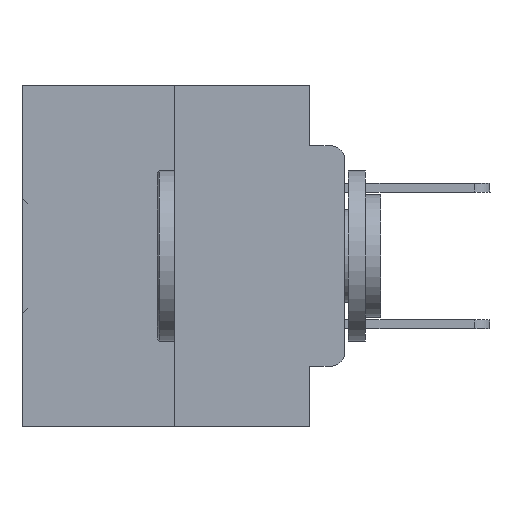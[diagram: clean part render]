
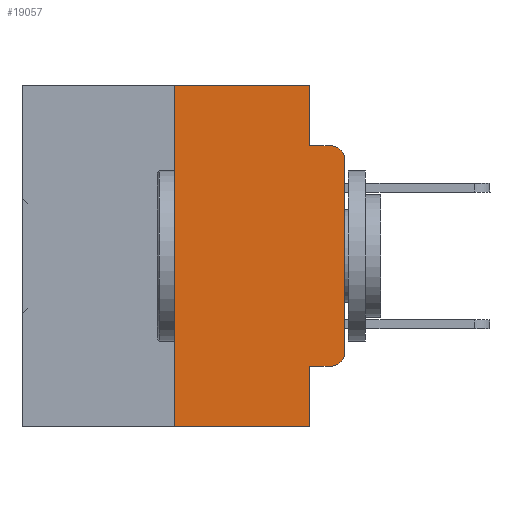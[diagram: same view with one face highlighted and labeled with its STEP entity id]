
A CAD part, left-side view. The second image highlights one B-rep face of the part: STEP entity #19057.
In plain terms, the highlighted planar face has unit normal (-1, 0, 0).
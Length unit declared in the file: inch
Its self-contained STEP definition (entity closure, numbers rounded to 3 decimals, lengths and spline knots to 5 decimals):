
#439 = CARTESIAN_POINT ( 'NONE',  ( 0., 0.25, -0.5 ) ) ;
#452 = VERTEX_POINT ( 'NONE', #18065 ) ;
#732 = LINE ( 'NONE', #26231, #28675 ) ;
#845 = DIRECTION ( 'NONE',  ( 0., 0., -1. ) ) ;
#938 = VERTEX_POINT ( 'NONE', #26433 ) ;
#1768 = EDGE_CURVE ( 'NONE', #10953, #12794, #3225, .T. ) ;
#1987 = ORIENTED_EDGE ( 'NONE', *, *, #24835, .T. ) ;
#2397 = CARTESIAN_POINT ( 'NONE',  ( 0., 0., -0.3915 ) ) ;
#2568 = VECTOR ( 'NONE', #14747, 39.37008 ) ;
#2595 = CARTESIAN_POINT ( 'NONE',  ( 0., 0.051, 0. ) ) ;
#3184 = LINE ( 'NONE', #2595, #34208 ) ;
#3225 = CIRCLE ( 'NONE', #23362, 0.02 ) ;
#3363 = ORIENTED_EDGE ( 'NONE', *, *, #1768, .T. ) ;
#3644 = EDGE_CURVE ( 'NONE', #938, #452, #19149, .T. ) ;
#4663 = EDGE_CURVE ( 'NONE', #452, #25880, #732, .T. ) ;
#4919 = DIRECTION ( 'NONE',  ( 0., 0., -1. ) ) ;
#5444 = EDGE_LOOP ( 'NONE', ( #15345, #13133, #7458, #34054, #29395, #20109, #1987, #13547, #15933, #3363 ) ) ;
#5489 = DIRECTION ( 'NONE',  ( 0., -1., 0. ) ) ;
#5684 = CARTESIAN_POINT ( 'NONE',  ( 0., 0.02, -0.1085 ) ) ;
#6436 = VECTOR ( 'NONE', #14248, 39.37008 ) ;
#6572 = CARTESIAN_POINT ( 'NONE',  ( 0., 0.02, -0.0885 ) ) ;
#7030 = VECTOR ( 'NONE', #5489, 39.37008 ) ;
#7458 = ORIENTED_EDGE ( 'NONE', *, *, #33987, .F. ) ;
#8885 = EDGE_CURVE ( 'NONE', #12794, #18100, #31506, .T. ) ;
#8930 = VERTEX_POINT ( 'NONE', #439 ) ;
#9142 = CIRCLE ( 'NONE', #29656, 0.02 ) ;
#10180 = CARTESIAN_POINT ( 'NONE',  ( 0., 0.051, -0.5 ) ) ;
#10953 = VERTEX_POINT ( 'NONE', #29867 ) ;
#11678 = DIRECTION ( 'NONE',  ( -1., 0., 0. ) ) ;
#11704 = VECTOR ( 'NONE', #27401, 39.37008 ) ;
#11819 = LINE ( 'NONE', #31291, #15779 ) ;
#12794 = VERTEX_POINT ( 'NONE', #2397 ) ;
#12837 = DIRECTION ( 'NONE',  ( -1., 0., 0. ) ) ;
#13133 = ORIENTED_EDGE ( 'NONE', *, *, #15701, .T. ) ;
#13547 = ORIENTED_EDGE ( 'NONE', *, *, #31042, .F. ) ;
#13794 = DIRECTION ( 'NONE',  ( 0., 0., 1. ) ) ;
#14150 = DIRECTION ( 'NONE',  ( 0., -1., 0. ) ) ;
#14248 = DIRECTION ( 'NONE',  ( 0., -1., 0. ) ) ;
#14505 = LINE ( 'NONE', #25138, #7030 ) ;
#14747 = DIRECTION ( 'NONE',  ( 0., 0., 1. ) ) ;
#15257 = VERTEX_POINT ( 'NONE', #6572 ) ;
#15345 = ORIENTED_EDGE ( 'NONE', *, *, #8885, .T. ) ;
#15427 = EDGE_CURVE ( 'NONE', #8930, #938, #20484, .T. ) ;
#15645 = DIRECTION ( 'NONE',  ( 0., 0., -1. ) ) ;
#15701 = EDGE_CURVE ( 'NONE', #18100, #15257, #9142, .T. ) ;
#15779 = VECTOR ( 'NONE', #14150, 39.37008 ) ;
#15933 = ORIENTED_EDGE ( 'NONE', *, *, #23652, .T. ) ;
#15951 = CARTESIAN_POINT ( 'NONE',  ( 0., 0.051, -0.0885 ) ) ;
#17008 = DIRECTION ( 'NONE',  ( 1., 0., 0. ) ) ;
#17283 = DIRECTION ( 'NONE',  ( 0., 0., -1. ) ) ;
#17371 = DIRECTION ( 'NONE',  ( 0., 0., -1. ) ) ;
#17821 = LINE ( 'NONE', #33832, #6436 ) ;
#18065 = CARTESIAN_POINT ( 'NONE',  ( 0., 0.051, 0. ) ) ;
#18100 = VERTEX_POINT ( 'NONE', #32677 ) ;
#19057 = ADVANCED_FACE ( 'NONE', ( #33786 ), #33944, .F. ) ;
#19149 = LINE ( 'NONE', #33002, #11704 ) ;
#20065 = CARTESIAN_POINT ( 'NONE',  ( 0., 0.051, -0.4115 ) ) ;
#20109 = ORIENTED_EDGE ( 'NONE', *, *, #15427, .F. ) ;
#20484 = LINE ( 'NONE', #30232, #28336 ) ;
#22487 = CARTESIAN_POINT ( 'NONE',  ( 0., 0.473, 0. ) ) ;
#23362 = AXIS2_PLACEMENT_3D ( 'NONE', #26730, #12837, #15645 ) ;
#23652 = EDGE_CURVE ( 'NONE', #29158, #10953, #11819, .T. ) ;
#24835 = EDGE_CURVE ( 'NONE', #8930, #31893, #17821, .T. ) ;
#25138 = CARTESIAN_POINT ( 'NONE',  ( 0., 0.051, -0.0885 ) ) ;
#25440 = CARTESIAN_POINT ( 'NONE',  ( 0., 0., 0. ) ) ;
#25880 = VERTEX_POINT ( 'NONE', #15951 ) ;
#26231 = CARTESIAN_POINT ( 'NONE',  ( 0., 0.051, 0. ) ) ;
#26433 = CARTESIAN_POINT ( 'NONE',  ( 0., 0.25, 0. ) ) ;
#26730 = CARTESIAN_POINT ( 'NONE',  ( 0., 0.02, -0.3915 ) ) ;
#27401 = DIRECTION ( 'NONE',  ( 0., -1., 0. ) ) ;
#28336 = VECTOR ( 'NONE', #13794, 39.37008 ) ;
#28675 = VECTOR ( 'NONE', #845, 39.37008 ) ;
#29158 = VERTEX_POINT ( 'NONE', #20065 ) ;
#29395 = ORIENTED_EDGE ( 'NONE', *, *, #3644, .F. ) ;
#29498 = AXIS2_PLACEMENT_3D ( 'NONE', #22487, #17008, #17371 ) ;
#29656 = AXIS2_PLACEMENT_3D ( 'NONE', #5684, #11678, #17283 ) ;
#29867 = CARTESIAN_POINT ( 'NONE',  ( 0., 0.02, -0.4115 ) ) ;
#30232 = CARTESIAN_POINT ( 'NONE',  ( 0., 0.25, 0. ) ) ;
#31042 = EDGE_CURVE ( 'NONE', #29158, #31893, #3184, .T. ) ;
#31291 = CARTESIAN_POINT ( 'NONE',  ( 0., 0.051, -0.4115 ) ) ;
#31506 = LINE ( 'NONE', #25440, #2568 ) ;
#31893 = VERTEX_POINT ( 'NONE', #10180 ) ;
#32677 = CARTESIAN_POINT ( 'NONE',  ( 0., 0., -0.1085 ) ) ;
#33002 = CARTESIAN_POINT ( 'NONE',  ( 0., 0.473, 0. ) ) ;
#33786 = FACE_OUTER_BOUND ( 'NONE', #5444, .T. ) ;
#33832 = CARTESIAN_POINT ( 'NONE',  ( 0., 0.473, -0.5 ) ) ;
#33944 = PLANE ( 'NONE',  #29498 ) ;
#33987 = EDGE_CURVE ( 'NONE', #25880, #15257, #14505, .T. ) ;
#34054 = ORIENTED_EDGE ( 'NONE', *, *, #4663, .F. ) ;
#34208 = VECTOR ( 'NONE', #4919, 39.37008 ) ;
